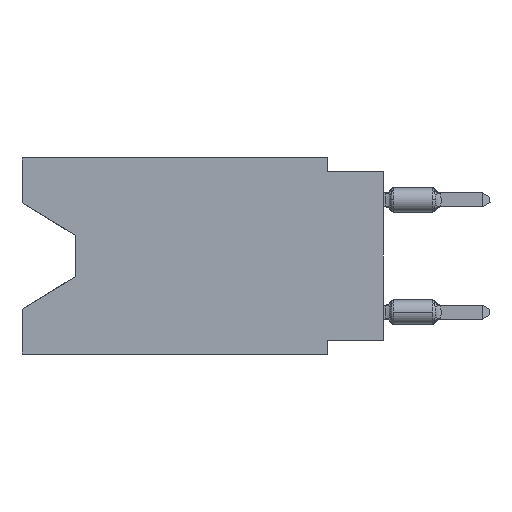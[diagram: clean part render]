
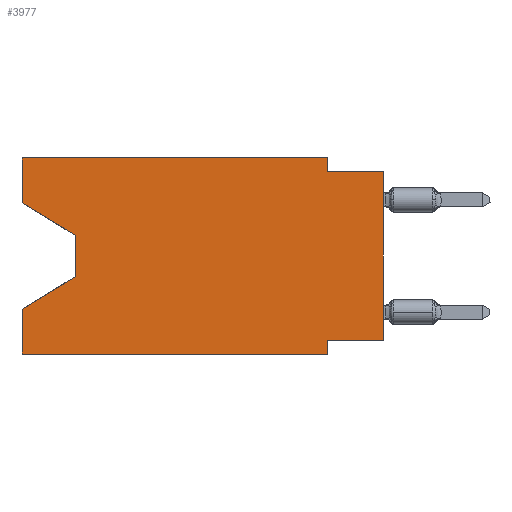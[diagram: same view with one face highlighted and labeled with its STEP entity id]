
A CAD part, left-side view. The second image highlights one B-rep face of the part: STEP entity #3977.
In plain terms, the highlighted planar face has unit normal (-1, 0, 0).
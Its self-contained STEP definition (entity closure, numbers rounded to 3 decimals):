
#835 = VECTOR ( 'NONE', #8884, 1000. ) ;
#841 = DIRECTION ( 'NONE',  ( 0., 0., 1. ) ) ;
#1106 = VECTOR ( 'NONE', #22239, 1000. ) ;
#1461 = CARTESIAN_POINT ( 'NONE',  ( 0., 16.383, -8.89 ) ) ;
#1674 = EDGE_LOOP ( 'NONE', ( #11449, #6026, #16310, #22154, #13615, #12611, #16513, #21472, #13551, #22611, #20879, #18905 ) ) ;
#1928 = EDGE_CURVE ( 'NONE', #25281, #23230, #20521, .T. ) ;
#3132 = VECTOR ( 'NONE', #841, 1000. ) ;
#3194 = CARTESIAN_POINT ( 'NONE',  ( 0., 13.97, -3.505 ) ) ;
#3318 = CARTESIAN_POINT ( 'NONE',  ( 0., 2.54, -8.255 ) ) ;
#3389 = VECTOR ( 'NONE', #16165, 1000. ) ;
#3668 = AXIS2_PLACEMENT_3D ( 'NONE', #25791, #12835, #17250 ) ;
#3977 = ADVANCED_FACE ( 'NONE', ( #11246 ), #8831, .F. ) ;
#4165 = EDGE_CURVE ( 'NONE', #26437, #27977, #11954, .T. ) ;
#4541 = VECTOR ( 'NONE', #21126, 1000. ) ;
#4857 = LINE ( 'NONE', #12999, #1106 ) ;
#4924 = DIRECTION ( 'NONE',  ( 0., 0., -1. ) ) ;
#5165 = VERTEX_POINT ( 'NONE', #8838 ) ;
#5268 = CARTESIAN_POINT ( 'NONE',  ( 0., 16.383, 0. ) ) ;
#5279 = CARTESIAN_POINT ( 'NONE',  ( 0., 16.383, -8.89 ) ) ;
#5703 = CARTESIAN_POINT ( 'NONE',  ( 0., 13.97, -5.385 ) ) ;
#6026 = ORIENTED_EDGE ( 'NONE', *, *, #11834, .T. ) ;
#6236 = CARTESIAN_POINT ( 'NONE',  ( 0., 2.54, 0. ) ) ;
#7113 = VECTOR ( 'NONE', #21353, 1000. ) ;
#7438 = CARTESIAN_POINT ( 'NONE',  ( 0., 2.54, -0.635 ) ) ;
#7611 = VERTEX_POINT ( 'NONE', #26574 ) ;
#7696 = VERTEX_POINT ( 'NONE', #3194 ) ;
#8459 = CARTESIAN_POINT ( 'NONE',  ( 0., 16.383, -6.852 ) ) ;
#8750 = VERTEX_POINT ( 'NONE', #6236 ) ;
#8757 = DIRECTION ( 'NONE',  ( 0., 0., 1. ) ) ;
#8831 = PLANE ( 'NONE',  #3668 ) ;
#8838 = CARTESIAN_POINT ( 'NONE',  ( 0., 0., -8.255 ) ) ;
#8884 = DIRECTION ( 'NONE',  ( 0., -0.855, -0.519 ) ) ;
#9210 = LINE ( 'NONE', #26588, #20356 ) ;
#9300 = LINE ( 'NONE', #18002, #835 ) ;
#10304 = EDGE_CURVE ( 'NONE', #5165, #26437, #20908, .T. ) ;
#10654 = EDGE_CURVE ( 'NONE', #8750, #23488, #9210, .T. ) ;
#11246 = FACE_OUTER_BOUND ( 'NONE', #1674, .T. ) ;
#11449 = ORIENTED_EDGE ( 'NONE', *, *, #23453, .T. ) ;
#11834 = EDGE_CURVE ( 'NONE', #7696, #7611, #22010, .T. ) ;
#11855 = EDGE_CURVE ( 'NONE', #12666, #20194, #17599, .T. ) ;
#11888 = LINE ( 'NONE', #24854, #3389 ) ;
#11954 = LINE ( 'NONE', #17957, #25053 ) ;
#12383 = LINE ( 'NONE', #22927, #7113 ) ;
#12611 = ORIENTED_EDGE ( 'NONE', *, *, #4165, .F. ) ;
#12666 = VERTEX_POINT ( 'NONE', #13776 ) ;
#12835 = DIRECTION ( 'NONE',  ( 1., 0., 0. ) ) ;
#12999 = CARTESIAN_POINT ( 'NONE',  ( 0., 16.383, 0. ) ) ;
#13489 = EDGE_CURVE ( 'NONE', #20194, #8750, #4857, .T. ) ;
#13551 = ORIENTED_EDGE ( 'NONE', *, *, #18958, .F. ) ;
#13615 = ORIENTED_EDGE ( 'NONE', *, *, #27719, .T. ) ;
#13776 = CARTESIAN_POINT ( 'NONE',  ( 0., 16.383, -2.038 ) ) ;
#13797 = EDGE_CURVE ( 'NONE', #7611, #23230, #20956, .T. ) ;
#15462 = CARTESIAN_POINT ( 'NONE',  ( 0., 13.97, -3.505 ) ) ;
#15917 = VECTOR ( 'NONE', #8757, 1000. ) ;
#16165 = DIRECTION ( 'NONE',  ( 0., 0., 1. ) ) ;
#16310 = ORIENTED_EDGE ( 'NONE', *, *, #13797, .T. ) ;
#16513 = ORIENTED_EDGE ( 'NONE', *, *, #10304, .F. ) ;
#16514 = CARTESIAN_POINT ( 'NONE',  ( 0., 0., -8.255 ) ) ;
#16751 = EDGE_CURVE ( 'NONE', #5165, #20293, #11888, .T. ) ;
#16822 = DIRECTION ( 'NONE',  ( 0., 0.855, -0.519 ) ) ;
#17250 = DIRECTION ( 'NONE',  ( 0., 0., -1. ) ) ;
#17599 = LINE ( 'NONE', #21869, #15917 ) ;
#17957 = CARTESIAN_POINT ( 'NONE',  ( 0., 2.54, -8.89 ) ) ;
#18002 = CARTESIAN_POINT ( 'NONE',  ( 0., 16.383, -2.038 ) ) ;
#18905 = ORIENTED_EDGE ( 'NONE', *, *, #11855, .F. ) ;
#18958 = EDGE_CURVE ( 'NONE', #23488, #20293, #12383, .T. ) ;
#19014 = VECTOR ( 'NONE', #23177, 1000. ) ;
#20194 = VERTEX_POINT ( 'NONE', #24344 ) ;
#20293 = VERTEX_POINT ( 'NONE', #24061 ) ;
#20356 = VECTOR ( 'NONE', #4924, 1000. ) ;
#20521 = LINE ( 'NONE', #5268, #3132 ) ;
#20879 = ORIENTED_EDGE ( 'NONE', *, *, #13489, .F. ) ;
#20908 = LINE ( 'NONE', #16514, #19014 ) ;
#20956 = LINE ( 'NONE', #5703, #26599 ) ;
#21126 = DIRECTION ( 'NONE',  ( 0., -1., 0. ) ) ;
#21353 = DIRECTION ( 'NONE',  ( 0., -1., 0. ) ) ;
#21472 = ORIENTED_EDGE ( 'NONE', *, *, #16751, .T. ) ;
#21869 = CARTESIAN_POINT ( 'NONE',  ( 0., 16.383, 0. ) ) ;
#22010 = LINE ( 'NONE', #15462, #26428 ) ;
#22154 = ORIENTED_EDGE ( 'NONE', *, *, #1928, .F. ) ;
#22239 = DIRECTION ( 'NONE',  ( 0., -1., 0. ) ) ;
#22611 = ORIENTED_EDGE ( 'NONE', *, *, #10654, .F. ) ;
#22913 = CARTESIAN_POINT ( 'NONE',  ( 0., 2.54, -8.89 ) ) ;
#22927 = CARTESIAN_POINT ( 'NONE',  ( 0., 0., -0.635 ) ) ;
#22978 = LINE ( 'NONE', #1461, #4541 ) ;
#23177 = DIRECTION ( 'NONE',  ( 0., 1., 0. ) ) ;
#23230 = VERTEX_POINT ( 'NONE', #8459 ) ;
#23453 = EDGE_CURVE ( 'NONE', #12666, #7696, #9300, .T. ) ;
#23488 = VERTEX_POINT ( 'NONE', #7438 ) ;
#24061 = CARTESIAN_POINT ( 'NONE',  ( 0., 0., -0.635 ) ) ;
#24141 = DIRECTION ( 'NONE',  ( 0., 0., -1. ) ) ;
#24344 = CARTESIAN_POINT ( 'NONE',  ( 0., 16.383, 0. ) ) ;
#24854 = CARTESIAN_POINT ( 'NONE',  ( 0., 0., 0. ) ) ;
#25053 = VECTOR ( 'NONE', #26636, 1000. ) ;
#25281 = VERTEX_POINT ( 'NONE', #5279 ) ;
#25791 = CARTESIAN_POINT ( 'NONE',  ( 0., 16.383, 0. ) ) ;
#26428 = VECTOR ( 'NONE', #24141, 1000. ) ;
#26437 = VERTEX_POINT ( 'NONE', #3318 ) ;
#26574 = CARTESIAN_POINT ( 'NONE',  ( 0., 13.97, -5.385 ) ) ;
#26588 = CARTESIAN_POINT ( 'NONE',  ( 0., 2.54, 0. ) ) ;
#26599 = VECTOR ( 'NONE', #16822, 1000. ) ;
#26636 = DIRECTION ( 'NONE',  ( 0., 0., -1. ) ) ;
#27719 = EDGE_CURVE ( 'NONE', #25281, #27977, #22978, .T. ) ;
#27977 = VERTEX_POINT ( 'NONE', #22913 ) ;
